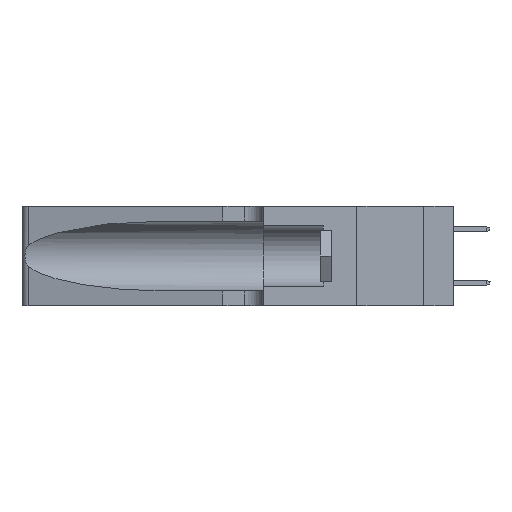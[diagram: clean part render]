
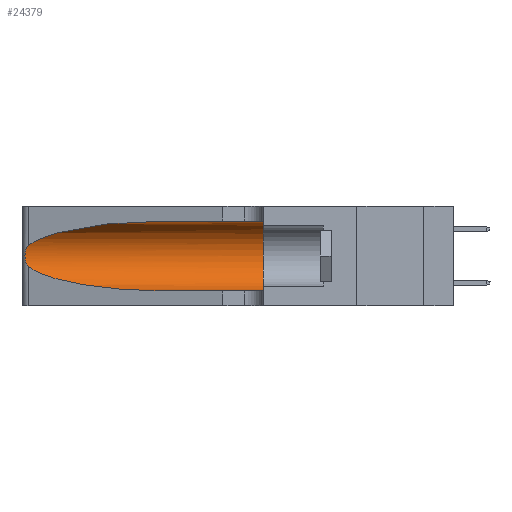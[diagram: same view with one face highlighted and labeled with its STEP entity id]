
A CAD part, left-side view. The second image highlights one B-rep face of the part: STEP entity #24379.
In plain terms, the highlighted cylindrical face has radius 3.308 mm (diameter 6.617 mm), a partial arc.
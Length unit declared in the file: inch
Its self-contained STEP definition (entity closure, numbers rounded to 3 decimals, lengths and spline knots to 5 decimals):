
#370 = CARTESIAN_POINT ( 'NONE',  ( 0.1305, 0.35, 0.31525 ) ) ;
#1425 = CARTESIAN_POINT ( 'NONE',  ( 0.1305, 0.72297, 0.05475 ) ) ;
#1576 = CARTESIAN_POINT ( 'NONE',  ( 0.18966, 0.96281, 0.05475 ) ) ;
#1871 = CARTESIAN_POINT ( 'NONE',  ( 0.25487, 1.22718, 0.22369 ) ) ;
#2015 = CARTESIAN_POINT ( 'NONE',  ( 0.25555, 1.22993, 0.14849 ) ) ;
#2073 = VERTEX_POINT ( 'NONE', #28658 ) ;
#2318 = DIRECTION ( 'NONE',  ( 0., 1., 0. ) ) ;
#2439 = ORIENTED_EDGE ( 'NONE', *, *, #9349, .F. ) ;
#4307 = CARTESIAN_POINT ( 'NONE',  ( 0.25789, 1.23486, 0.15765 ) ) ;
#4479 = VERTEX_POINT ( 'NONE', #370 ) ;
#4535 = CARTESIAN_POINT ( 'NONE',  ( 0.1305, 1.61858, 0.05475 ) ) ;
#4819 = DIRECTION ( 'NONE',  ( 0., 0., -1. ) ) ;
#5022 = CIRCLE ( 'NONE', #10916, 0.13025 ) ;
#5440 = ORIENTED_EDGE ( 'NONE', *, *, #24660, .T. ) ;
#6117 =( BOUNDED_CURVE ( )  B_SPLINE_CURVE ( 3, ( #15543, #10944, #13222, #29657 ),
 .UNSPECIFIED., .F., .T. ) 
 B_SPLINE_CURVE_WITH_KNOTS ( ( 4, 4 ),
 ( 1.5708, 2.84003 ),
 .UNSPECIFIED. ) 
 CURVE ( )  GEOMETRIC_REPRESENTATION_ITEM ( )  RATIONAL_B_SPLINE_CURVE ( ( 1., 0.87, 0.87, 1. ) ) 
 REPRESENTATION_ITEM ( '' )  );
#6431 = CARTESIAN_POINT ( 'NONE',  ( 0.25787, 1.23484, 0.2124 ) ) ;
#6755 = CARTESIAN_POINT ( 'NONE',  ( 0.25639, 1.23184, 0.21858 ) ) ;
#6892 = CARTESIAN_POINT ( 'NONE',  ( 0.1305, 0.35, 0.185 ) ) ;
#7357 = AXIS2_PLACEMENT_3D ( 'NONE', #18774, #20753, #4819 ) ;
#8681 = DIRECTION ( 'NONE',  ( 0., -1., 0. ) ) ;
#9069 = CARTESIAN_POINT ( 'NONE',  ( 0.25555, 1.22994, 0.2215 ) ) ;
#9349 = EDGE_CURVE ( 'NONE', #15975, #4479, #9843, .T. ) ;
#9780 = VECTOR ( 'NONE', #8681, 39.37008 ) ;
#9804 = EDGE_CURVE ( 'NONE', #16875, #30108, #29564, .T. ) ;
#9843 = LINE ( 'NONE', #19188, #21466 ) ;
#10101 = ORIENTED_EDGE ( 'NONE', *, *, #9804, .T. ) ;
#10916 = AXIS2_PLACEMENT_3D ( 'NONE', #6892, #2318, #29770 ) ;
#10944 = CARTESIAN_POINT ( 'NONE',  ( 0.18966, 0.96281, 0.31525 ) ) ;
#11213 = CARTESIAN_POINT ( 'NONE',  ( 0.26018, 1.23835, 0.19895 ) ) ;
#12035 = ORIENTED_EDGE ( 'NONE', *, *, #16211, .F. ) ;
#12414 = CARTESIAN_POINT ( 'NONE',  ( 0.25487, 1.22718, 0.22369 ) ) ;
#13001 = EDGE_CURVE ( 'NONE', #29869, #2073, #14919, .T. ) ;
#13222 = CARTESIAN_POINT ( 'NONE',  ( 0.2373, 1.15595, 0.28018 ) ) ;
#14184 = FACE_OUTER_BOUND ( 'NONE', #25970, .T. ) ;
#14214 = CARTESIAN_POINT ( 'NONE',  ( 0.1305, 0.35, 0.05475 ) ) ;
#14919 = B_SPLINE_CURVE_WITH_KNOTS ( 'NONE', 3,
 ( #1871, #9069, #6755, #6431, #27360, #11213, #20528, #29775, #16105, #25249, #4307, #22952, #2015, #29933 ),
 .UNSPECIFIED., .F., .F.,
 ( 4, 2, 2, 2, 2, 2, 4 ),
 ( 0., 0.00027, 0.00053, 0.00107, 0.0016, 0.00187, 0.00214 ),
 .UNSPECIFIED. ) ;
#15543 = CARTESIAN_POINT ( 'NONE',  ( 0.1305, 0.72297, 0.31525 ) ) ;
#15975 = VERTEX_POINT ( 'NONE', #30127 ) ;
#16105 = CARTESIAN_POINT ( 'NONE',  ( 0.26017, 1.23833, 0.17102 ) ) ;
#16211 = EDGE_CURVE ( 'NONE', #4479, #30108, #5022, .T. ) ;
#16875 = VERTEX_POINT ( 'NONE', #19633 ) ;
#17941 = EDGE_CURVE ( 'NONE', #2073, #16875, #24878, .T. ) ;
#18774 = CARTESIAN_POINT ( 'NONE',  ( 0.1305, 1.61858, 0.185 ) ) ;
#19188 = CARTESIAN_POINT ( 'NONE',  ( 0.1305, 1.61858, 0.31525 ) ) ;
#19633 = CARTESIAN_POINT ( 'NONE',  ( 0.1305, 0.72297, 0.05475 ) ) ;
#20528 = CARTESIAN_POINT ( 'NONE',  ( 0.26075, 1.23896, 0.19203 ) ) ;
#20753 = DIRECTION ( 'NONE',  ( 0., -1., 0. ) ) ;
#21466 = VECTOR ( 'NONE', #26171, 39.37008 ) ;
#22363 = CARTESIAN_POINT ( 'NONE',  ( 0.2373, 1.15595, 0.08982 ) ) ;
#22952 = CARTESIAN_POINT ( 'NONE',  ( 0.25639, 1.23186, 0.15144 ) ) ;
#23560 = ORIENTED_EDGE ( 'NONE', *, *, #13001, .T. ) ;
#24379 = ADVANCED_FACE ( 'NONE', ( #14184 ), #27590, .F. ) ;
#24660 = EDGE_CURVE ( 'NONE', #15975, #29869, #6117, .T. ) ;
#24878 =( BOUNDED_CURVE ( )  B_SPLINE_CURVE ( 3, ( #26909, #22363, #1576, #1425 ),
 .UNSPECIFIED., .F., .T. ) 
 B_SPLINE_CURVE_WITH_KNOTS ( ( 4, 4 ),
 ( 3.44316, 4.71239 ),
 .UNSPECIFIED. ) 
 CURVE ( )  GEOMETRIC_REPRESENTATION_ITEM ( )  RATIONAL_B_SPLINE_CURVE ( ( 1., 0.87, 0.87, 1. ) ) 
 REPRESENTATION_ITEM ( '' )  );
#25249 = CARTESIAN_POINT ( 'NONE',  ( 0.25856, 1.23593, 0.16098 ) ) ;
#25970 = EDGE_LOOP ( 'NONE', ( #5440, #23560, #28547, #10101, #12035, #2439 ) ) ;
#26171 = DIRECTION ( 'NONE',  ( 0., -1., 0. ) ) ;
#26909 = CARTESIAN_POINT ( 'NONE',  ( 0.25487, 1.22718, 0.14631 ) ) ;
#27360 = CARTESIAN_POINT ( 'NONE',  ( 0.25854, 1.2359, 0.20912 ) ) ;
#27590 = CYLINDRICAL_SURFACE ( 'NONE', #7357, 0.13025 ) ;
#28547 = ORIENTED_EDGE ( 'NONE', *, *, #17941, .T. ) ;
#28658 = CARTESIAN_POINT ( 'NONE',  ( 0.25487, 1.22718, 0.14631 ) ) ;
#29564 = LINE ( 'NONE', #4535, #9780 ) ;
#29657 = CARTESIAN_POINT ( 'NONE',  ( 0.25487, 1.22718, 0.22369 ) ) ;
#29770 = DIRECTION ( 'NONE',  ( 0., 0., 1. ) ) ;
#29775 = CARTESIAN_POINT ( 'NONE',  ( 0.26075, 1.23896, 0.178 ) ) ;
#29869 = VERTEX_POINT ( 'NONE', #12414 ) ;
#29933 = CARTESIAN_POINT ( 'NONE',  ( 0.25487, 1.22718, 0.14631 ) ) ;
#30108 = VERTEX_POINT ( 'NONE', #14214 ) ;
#30127 = CARTESIAN_POINT ( 'NONE',  ( 0.1305, 0.72297, 0.31525 ) ) ;
